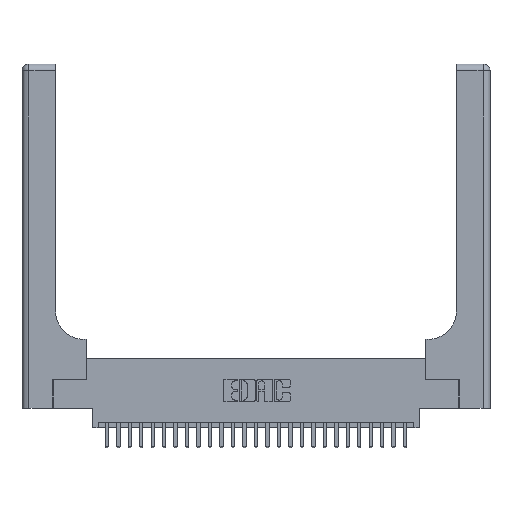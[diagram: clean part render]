
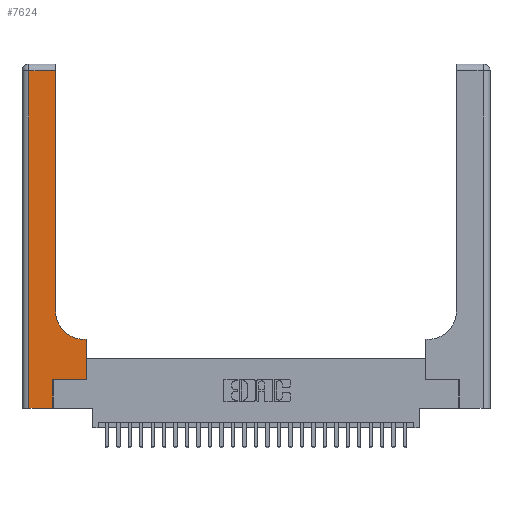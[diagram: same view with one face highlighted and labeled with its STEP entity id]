
A CAD part, top view. The second image highlights one B-rep face of the part: STEP entity #7624.
In plain terms, the highlighted planar face has unit normal (0, 0, 1).
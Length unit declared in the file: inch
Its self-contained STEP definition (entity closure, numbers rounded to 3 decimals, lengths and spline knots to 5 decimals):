
#324 = EDGE_CURVE ( 'NONE', #24373, #1480, #19403, .T. ) ;
#374 = EDGE_CURVE ( 'NONE', #15207, #2683, #17313, .T. ) ;
#807 = LINE ( 'NONE', #21665, #23712 ) ;
#1480 = VERTEX_POINT ( 'NONE', #19759 ) ;
#1890 = EDGE_CURVE ( 'NONE', #12130, #13260, #14409, .T. ) ;
#2097 = VERTEX_POINT ( 'NONE', #15735 ) ;
#2129 = CARTESIAN_POINT ( 'NONE',  ( 0.269, 0., 0.37 ) ) ;
#2477 = CARTESIAN_POINT ( 'NONE',  ( 0.2915, 0.85, 0.37 ) ) ;
#2683 = VERTEX_POINT ( 'NONE', #20181 ) ;
#2851 = FACE_OUTER_BOUND ( 'NONE', #17480, .T. ) ;
#3229 = VERTEX_POINT ( 'NONE', #24163 ) ;
#3230 = CARTESIAN_POINT ( 'NONE',  ( 0.5585, 0.6, 0.37 ) ) ;
#3233 = VECTOR ( 'NONE', #13403, 39.37008 ) ;
#3313 = EDGE_CURVE ( 'NONE', #2097, #12130, #10550, .T. ) ;
#3737 = ORIENTED_EDGE ( 'NONE', *, *, #3313, .T. ) ;
#4545 = AXIS2_PLACEMENT_3D ( 'NONE', #7099, #22612, #9327 ) ;
#6101 = DIRECTION ( 'NONE',  ( 1., 0., 0. ) ) ;
#6195 = VECTOR ( 'NONE', #15595, 39.37008 ) ;
#6537 = ORIENTED_EDGE ( 'NONE', *, *, #1890, .T. ) ;
#6657 = CARTESIAN_POINT ( 'NONE',  ( 0.5415, 0.85, 0.37 ) ) ;
#7051 = CARTESIAN_POINT ( 'NONE',  ( 0.06, 3., 0.37 ) ) ;
#7099 = CARTESIAN_POINT ( 'NONE',  ( 0., 3., 0.37 ) ) ;
#7232 = ORIENTED_EDGE ( 'NONE', *, *, #20124, .T. ) ;
#7624 = ADVANCED_FACE ( 'NONE', ( #2851 ), #15833, .F. ) ;
#8015 = VECTOR ( 'NONE', #10551, 39.37008 ) ;
#8280 = VECTOR ( 'NONE', #18193, 39.37008 ) ;
#8632 = EDGE_CURVE ( 'NONE', #26604, #24373, #19135, .T. ) ;
#8642 = CIRCLE ( 'NONE', #18958, 0.25 ) ;
#8881 = DIRECTION ( 'NONE',  ( 1., 0., 0. ) ) ;
#8965 = CARTESIAN_POINT ( 'NONE',  ( 0., 0., 0.37 ) ) ;
#9327 = DIRECTION ( 'NONE',  ( -1., 0., 0. ) ) ;
#9650 = VECTOR ( 'NONE', #27064, 39.37008 ) ;
#10550 = LINE ( 'NONE', #8965, #3233 ) ;
#10551 = DIRECTION ( 'NONE',  ( 0., 1., 0. ) ) ;
#10788 = CARTESIAN_POINT ( 'NONE',  ( 0.5585, 0.25, 0.37 ) ) ;
#11393 = ORIENTED_EDGE ( 'NONE', *, *, #324, .T. ) ;
#12130 = VERTEX_POINT ( 'NONE', #2129 ) ;
#12289 = LINE ( 'NONE', #7051, #23408 ) ;
#13260 = VERTEX_POINT ( 'NONE', #24859 ) ;
#13403 = DIRECTION ( 'NONE',  ( 1., 0., 0. ) ) ;
#13716 = VECTOR ( 'NONE', #17205, 39.37008 ) ;
#13723 = CARTESIAN_POINT ( 'NONE',  ( 0., 2.94, 0.37 ) ) ;
#13749 = EDGE_CURVE ( 'NONE', #1480, #15207, #8642, .T. ) ;
#14133 = ORIENTED_EDGE ( 'NONE', *, *, #18653, .T. ) ;
#14409 = LINE ( 'NONE', #14941, #13716 ) ;
#14941 = CARTESIAN_POINT ( 'NONE',  ( 0.269, 0., 0.37 ) ) ;
#15071 = EDGE_CURVE ( 'NONE', #2683, #3229, #21475, .T. ) ;
#15207 = VERTEX_POINT ( 'NONE', #2477 ) ;
#15595 = DIRECTION ( 'NONE',  ( 0., 1., 0. ) ) ;
#15624 = CARTESIAN_POINT ( 'NONE',  ( 0.2915, 3., 0.37 ) ) ;
#15735 = CARTESIAN_POINT ( 'NONE',  ( 0.06, 0., 0.37 ) ) ;
#15833 = PLANE ( 'NONE',  #4545 ) ;
#16074 = DIRECTION ( 'NONE',  ( 0., -1., 0. ) ) ;
#16595 = ORIENTED_EDGE ( 'NONE', *, *, #8632, .T. ) ;
#17205 = DIRECTION ( 'NONE',  ( 0., 1., 0. ) ) ;
#17313 = LINE ( 'NONE', #15624, #6195 ) ;
#17480 = EDGE_LOOP ( 'NONE', ( #22802, #26245, #14133, #3737, #6537, #7232, #16595, #11393, #23869 ) ) ;
#17714 = CARTESIAN_POINT ( 'NONE',  ( 0.2915, 0.6, 0.37 ) ) ;
#18193 = DIRECTION ( 'NONE',  ( -1., 0., 0. ) ) ;
#18653 = EDGE_CURVE ( 'NONE', #3229, #2097, #12289, .T. ) ;
#18958 = AXIS2_PLACEMENT_3D ( 'NONE', #6657, #22176, #8881 ) ;
#19135 = LINE ( 'NONE', #26011, #8015 ) ;
#19403 = LINE ( 'NONE', #17714, #8280 ) ;
#19759 = CARTESIAN_POINT ( 'NONE',  ( 0.5415, 0.6, 0.37 ) ) ;
#20124 = EDGE_CURVE ( 'NONE', #13260, #26604, #807, .T. ) ;
#20181 = CARTESIAN_POINT ( 'NONE',  ( 0.2915, 2.94, 0.37 ) ) ;
#21475 = LINE ( 'NONE', #13723, #9650 ) ;
#21665 = CARTESIAN_POINT ( 'NONE',  ( 0.269, 0.25, 0.37 ) ) ;
#22176 = DIRECTION ( 'NONE',  ( 0., 0., -1. ) ) ;
#22612 = DIRECTION ( 'NONE',  ( 0., 0., -1. ) ) ;
#22802 = ORIENTED_EDGE ( 'NONE', *, *, #374, .T. ) ;
#23408 = VECTOR ( 'NONE', #16074, 39.37008 ) ;
#23712 = VECTOR ( 'NONE', #6101, 39.37008 ) ;
#23869 = ORIENTED_EDGE ( 'NONE', *, *, #13749, .T. ) ;
#24163 = CARTESIAN_POINT ( 'NONE',  ( 0.06, 2.94, 0.37 ) ) ;
#24373 = VERTEX_POINT ( 'NONE', #3230 ) ;
#24859 = CARTESIAN_POINT ( 'NONE',  ( 0.269, 0.25, 0.37 ) ) ;
#26011 = CARTESIAN_POINT ( 'NONE',  ( 0.5585, 0.25, 0.37 ) ) ;
#26245 = ORIENTED_EDGE ( 'NONE', *, *, #15071, .T. ) ;
#26604 = VERTEX_POINT ( 'NONE', #10788 ) ;
#27064 = DIRECTION ( 'NONE',  ( -1., 0., 0. ) ) ;
